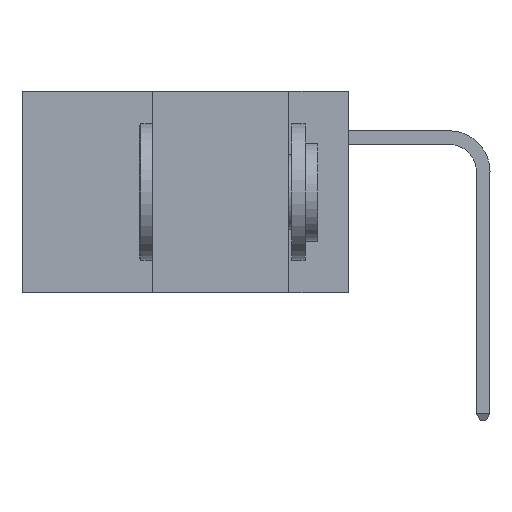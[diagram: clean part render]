
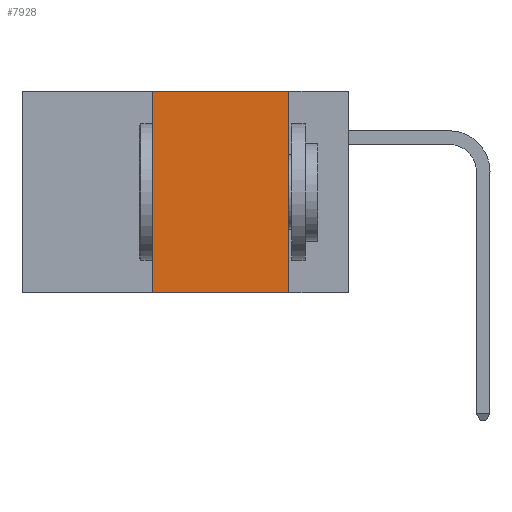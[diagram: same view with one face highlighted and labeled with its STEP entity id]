
A CAD part, left-side view. The second image highlights one B-rep face of the part: STEP entity #7928.
In plain terms, the highlighted planar face has unit normal (-1, 0, 0).
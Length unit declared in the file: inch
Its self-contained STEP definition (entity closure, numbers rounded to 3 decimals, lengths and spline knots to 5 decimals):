
#788 = EDGE_LOOP ( 'NONE', ( #17618, #7773, #14618, #22560 ) ) ;
#1959 = EDGE_CURVE ( 'NONE', #16807, #10126, #19020, .T. ) ;
#2798 = LINE ( 'NONE', #5577, #6488 ) ;
#5577 = CARTESIAN_POINT ( 'NONE',  ( 0., 0.6, -0.37 ) ) ;
#5641 = EDGE_CURVE ( 'NONE', #16807, #22363, #2798, .T. ) ;
#6283 = PLANE ( 'NONE',  #10897 ) ;
#6488 = VECTOR ( 'NONE', #19908, 39.37008 ) ;
#7459 = CARTESIAN_POINT ( 'NONE',  ( 0., 0.11, 0. ) ) ;
#7477 = VERTEX_POINT ( 'NONE', #10514 ) ;
#7773 = ORIENTED_EDGE ( 'NONE', *, *, #11436, .F. ) ;
#7928 = ADVANCED_FACE ( 'NONE', ( #22804 ), #6283, .F. ) ;
#8109 = CARTESIAN_POINT ( 'NONE',  ( 0., 0.11, -0.37 ) ) ;
#8679 = CARTESIAN_POINT ( 'NONE',  ( 0., 0.6, 0. ) ) ;
#9206 = CARTESIAN_POINT ( 'NONE',  ( 0., 0.36, 0. ) ) ;
#9209 = DIRECTION ( 'NONE',  ( 0., 0., 1. ) ) ;
#9515 = VECTOR ( 'NONE', #9209, 39.37008 ) ;
#9939 = DIRECTION ( 'NONE',  ( 0., 0., -1. ) ) ;
#10126 = VERTEX_POINT ( 'NONE', #12251 ) ;
#10514 = CARTESIAN_POINT ( 'NONE',  ( 0., 0.11, 0. ) ) ;
#10897 = AXIS2_PLACEMENT_3D ( 'NONE', #18838, #20578, #9939 ) ;
#11141 = DIRECTION ( 'NONE',  ( 0., 0., -1. ) ) ;
#11436 = EDGE_CURVE ( 'NONE', #10126, #7477, #14720, .T. ) ;
#12251 = CARTESIAN_POINT ( 'NONE',  ( 0., 0.36, 0. ) ) ;
#14055 = DIRECTION ( 'NONE',  ( 0., -1., 0. ) ) ;
#14618 = ORIENTED_EDGE ( 'NONE', *, *, #1959, .F. ) ;
#14720 = LINE ( 'NONE', #8679, #22920 ) ;
#14935 = CARTESIAN_POINT ( 'NONE',  ( 0., 0.36, -0.37 ) ) ;
#15719 = VECTOR ( 'NONE', #11141, 39.37008 ) ;
#16807 = VERTEX_POINT ( 'NONE', #14935 ) ;
#17618 = ORIENTED_EDGE ( 'NONE', *, *, #22778, .F. ) ;
#18838 = CARTESIAN_POINT ( 'NONE',  ( 0., 0.6, 0. ) ) ;
#19020 = LINE ( 'NONE', #9206, #9515 ) ;
#19908 = DIRECTION ( 'NONE',  ( 0., -1., 0. ) ) ;
#20403 = LINE ( 'NONE', #7459, #15719 ) ;
#20578 = DIRECTION ( 'NONE',  ( 1., 0., 0. ) ) ;
#22363 = VERTEX_POINT ( 'NONE', #8109 ) ;
#22560 = ORIENTED_EDGE ( 'NONE', *, *, #5641, .T. ) ;
#22778 = EDGE_CURVE ( 'NONE', #7477, #22363, #20403, .T. ) ;
#22804 = FACE_OUTER_BOUND ( 'NONE', #788, .T. ) ;
#22920 = VECTOR ( 'NONE', #14055, 39.37008 ) ;
